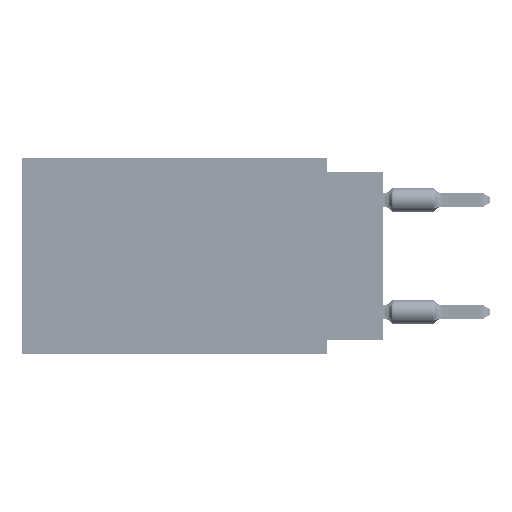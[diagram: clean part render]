
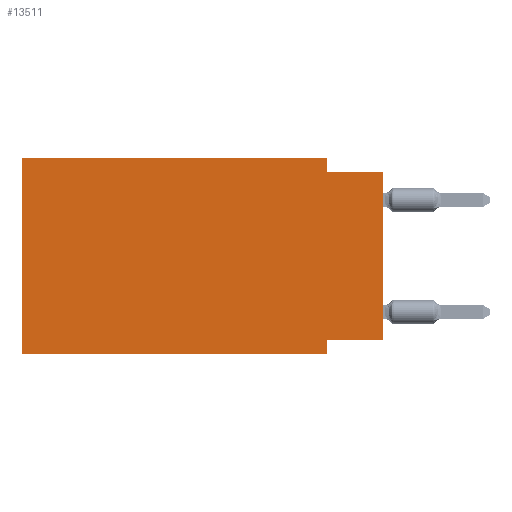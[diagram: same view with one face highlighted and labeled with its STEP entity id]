
A CAD part, left-side view. The second image highlights one B-rep face of the part: STEP entity #13511.
In plain terms, the highlighted planar face has unit normal (-1, 0, 0).
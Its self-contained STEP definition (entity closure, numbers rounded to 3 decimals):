
#378 = CARTESIAN_POINT ( 'NONE',  ( 0., 0., -8.255 ) ) ;
#503 = ORIENTED_EDGE ( 'NONE', *, *, #6276, .F. ) ;
#734 = CARTESIAN_POINT ( 'NONE',  ( 0., 0., -0.635 ) ) ;
#1790 = ORIENTED_EDGE ( 'NONE', *, *, #39785, .F. ) ;
#2348 = LINE ( 'NONE', #6913, #60904 ) ;
#3818 = VERTEX_POINT ( 'NONE', #39144 ) ;
#3885 = DIRECTION ( 'NONE',  ( 0., 0., -1. ) ) ;
#4242 = FACE_OUTER_BOUND ( 'NONE', #30322, .T. ) ;
#4253 = VECTOR ( 'NONE', #43462, 1000. ) ;
#5700 = CARTESIAN_POINT ( 'NONE',  ( 0., 2.54, -8.89 ) ) ;
#6276 = EDGE_CURVE ( 'NONE', #29766, #13293, #26050, .T. ) ;
#6913 = CARTESIAN_POINT ( 'NONE',  ( 0., 0., 0. ) ) ;
#9668 = ORIENTED_EDGE ( 'NONE', *, *, #13613, .F. ) ;
#9773 = DIRECTION ( 'NONE',  ( 0., -1., 0. ) ) ;
#10808 = ORIENTED_EDGE ( 'NONE', *, *, #40096, .T. ) ;
#11262 = LINE ( 'NONE', #31960, #26403 ) ;
#11954 = CARTESIAN_POINT ( 'NONE',  ( 0., 16.383, 0. ) ) ;
#13228 = DIRECTION ( 'NONE',  ( 0., 0., 1. ) ) ;
#13293 = VERTEX_POINT ( 'NONE', #734 ) ;
#13511 = ADVANCED_FACE ( 'NONE', ( #4242 ), #25957, .F. ) ;
#13613 = EDGE_CURVE ( 'NONE', #23601, #37082, #17186, .T. ) ;
#17186 = LINE ( 'NONE', #27033, #4253 ) ;
#17787 = DIRECTION ( 'NONE',  ( 0., 0., 1. ) ) ;
#18490 = CARTESIAN_POINT ( 'NONE',  ( 0., 16.383, 0. ) ) ;
#19828 = VECTOR ( 'NONE', #35565, 1000. ) ;
#20038 = LINE ( 'NONE', #57861, #45348 ) ;
#20702 = CARTESIAN_POINT ( 'NONE',  ( 0., 16.383, 0. ) ) ;
#20710 = VECTOR ( 'NONE', #20785, 1000. ) ;
#20785 = DIRECTION ( 'NONE',  ( 0., -1., 0. ) ) ;
#22189 = AXIS2_PLACEMENT_3D ( 'NONE', #20702, #36475, #3885 ) ;
#22204 = VERTEX_POINT ( 'NONE', #378 ) ;
#22725 = LINE ( 'NONE', #18490, #60027 ) ;
#23601 = VERTEX_POINT ( 'NONE', #67700 ) ;
#25957 = PLANE ( 'NONE',  #22189 ) ;
#26050 = LINE ( 'NONE', #26413, #20710 ) ;
#26403 = VECTOR ( 'NONE', #63454, 1000. ) ;
#26413 = CARTESIAN_POINT ( 'NONE',  ( 0., 0., -0.635 ) ) ;
#26563 = CARTESIAN_POINT ( 'NONE',  ( 0., 2.54, -0.635 ) ) ;
#27033 = CARTESIAN_POINT ( 'NONE',  ( 0., 2.54, -8.89 ) ) ;
#27554 = VECTOR ( 'NONE', #9773, 1000. ) ;
#29766 = VERTEX_POINT ( 'NONE', #26563 ) ;
#30322 = EDGE_LOOP ( 'NONE', ( #33960, #503, #69241, #30877, #54550, #10808, #9668, #1790 ) ) ;
#30877 = ORIENTED_EDGE ( 'NONE', *, *, #67060, .F. ) ;
#31254 = CARTESIAN_POINT ( 'NONE',  ( 0., 2.54, 0. ) ) ;
#31960 = CARTESIAN_POINT ( 'NONE',  ( 0., 0., -8.255 ) ) ;
#33806 = EDGE_CURVE ( 'NONE', #53659, #29766, #46388, .T. ) ;
#33960 = ORIENTED_EDGE ( 'NONE', *, *, #43337, .T. ) ;
#35565 = DIRECTION ( 'NONE',  ( 0., 0., -1. ) ) ;
#36475 = DIRECTION ( 'NONE',  ( 1., 0., 0. ) ) ;
#37082 = VERTEX_POINT ( 'NONE', #5700 ) ;
#39144 = CARTESIAN_POINT ( 'NONE',  ( 0., 16.383, -8.89 ) ) ;
#39785 = EDGE_CURVE ( 'NONE', #22204, #23601, #11262, .T. ) ;
#40096 = EDGE_CURVE ( 'NONE', #3818, #37082, #51495, .T. ) ;
#41654 = CARTESIAN_POINT ( 'NONE',  ( 0., 16.383, -8.89 ) ) ;
#43337 = EDGE_CURVE ( 'NONE', #22204, #13293, #2348, .T. ) ;
#43462 = DIRECTION ( 'NONE',  ( 0., 0., -1. ) ) ;
#45348 = VECTOR ( 'NONE', #52610, 1000. ) ;
#46388 = LINE ( 'NONE', #56922, #19828 ) ;
#51495 = LINE ( 'NONE', #41654, #27554 ) ;
#52610 = DIRECTION ( 'NONE',  ( 0., -1., 0. ) ) ;
#53659 = VERTEX_POINT ( 'NONE', #31254 ) ;
#54550 = ORIENTED_EDGE ( 'NONE', *, *, #67706, .F. ) ;
#56922 = CARTESIAN_POINT ( 'NONE',  ( 0., 2.54, 0. ) ) ;
#57861 = CARTESIAN_POINT ( 'NONE',  ( 0., 16.383, 0. ) ) ;
#60027 = VECTOR ( 'NONE', #13228, 1000. ) ;
#60904 = VECTOR ( 'NONE', #17787, 1000. ) ;
#63454 = DIRECTION ( 'NONE',  ( 0., 1., 0. ) ) ;
#67060 = EDGE_CURVE ( 'NONE', #68378, #53659, #20038, .T. ) ;
#67700 = CARTESIAN_POINT ( 'NONE',  ( 0., 2.54, -8.255 ) ) ;
#67706 = EDGE_CURVE ( 'NONE', #3818, #68378, #22725, .T. ) ;
#68378 = VERTEX_POINT ( 'NONE', #11954 ) ;
#69241 = ORIENTED_EDGE ( 'NONE', *, *, #33806, .F. ) ;
